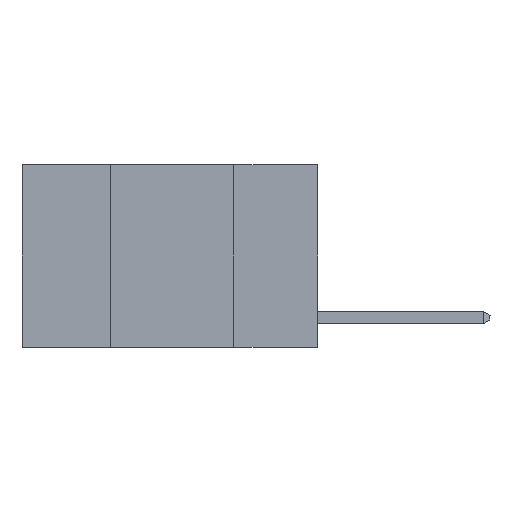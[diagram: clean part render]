
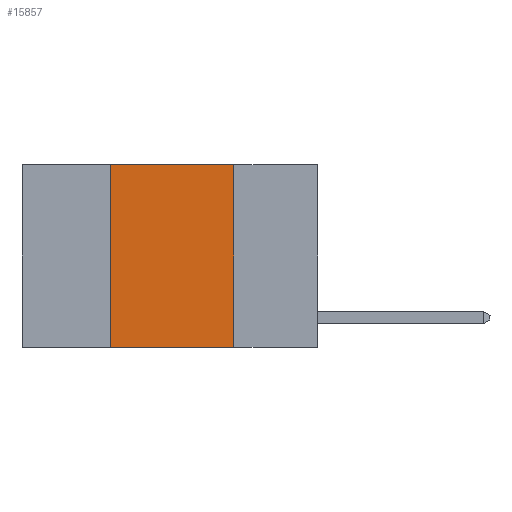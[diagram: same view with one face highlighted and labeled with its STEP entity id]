
A CAD part, left-side view. The second image highlights one B-rep face of the part: STEP entity #15857.
In plain terms, the highlighted planar face has unit normal (-1, 0, 0).
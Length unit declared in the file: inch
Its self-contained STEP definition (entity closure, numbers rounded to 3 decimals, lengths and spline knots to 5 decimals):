
#527 = FACE_OUTER_BOUND ( 'NONE', #12159, .T. ) ;
#928 = CARTESIAN_POINT ( 'NONE',  ( 0., 0.42, 0. ) ) ;
#1466 = VERTEX_POINT ( 'NONE', #21870 ) ;
#1476 = CARTESIAN_POINT ( 'NONE',  ( 0., 0.6, -0.37 ) ) ;
#1967 = VERTEX_POINT ( 'NONE', #24077 ) ;
#2682 = EDGE_CURVE ( 'NONE', #24479, #22064, #15013, .T. ) ;
#3091 = PLANE ( 'NONE',  #19471 ) ;
#3230 = DIRECTION ( 'NONE',  ( 0., 0., -1. ) ) ;
#3296 = VECTOR ( 'NONE', #20088, 39.37008 ) ;
#3658 = DIRECTION ( 'NONE',  ( 0., -1., 0. ) ) ;
#3993 = ORIENTED_EDGE ( 'NONE', *, *, #6999, .T. ) ;
#4603 = EDGE_CURVE ( 'NONE', #1967, #1466, #7291, .T. ) ;
#6799 = CARTESIAN_POINT ( 'NONE',  ( 0., 0.6, 0. ) ) ;
#6893 = DIRECTION ( 'NONE',  ( 1., 0., 0. ) ) ;
#6999 = EDGE_CURVE ( 'NONE', #1967, #22064, #16315, .T. ) ;
#7041 = CARTESIAN_POINT ( 'NONE',  ( 0., 0.17, 0. ) ) ;
#7110 = VECTOR ( 'NONE', #3230, 39.37008 ) ;
#7291 = LINE ( 'NONE', #928, #3296 ) ;
#8667 = VECTOR ( 'NONE', #3658, 39.37008 ) ;
#11179 = ORIENTED_EDGE ( 'NONE', *, *, #4603, .F. ) ;
#11641 = LINE ( 'NONE', #14410, #16242 ) ;
#12159 = EDGE_LOOP ( 'NONE', ( #19335, #12202, #11179, #3993 ) ) ;
#12202 = ORIENTED_EDGE ( 'NONE', *, *, #17796, .F. ) ;
#14410 = CARTESIAN_POINT ( 'NONE',  ( 0., 0.6, 0. ) ) ;
#15013 = LINE ( 'NONE', #15169, #7110 ) ;
#15169 = CARTESIAN_POINT ( 'NONE',  ( 0., 0.17, 0. ) ) ;
#15857 = ADVANCED_FACE ( 'NONE', ( #527 ), #3091, .F. ) ;
#16242 = VECTOR ( 'NONE', #22488, 39.37008 ) ;
#16315 = LINE ( 'NONE', #1476, #8667 ) ;
#17796 = EDGE_CURVE ( 'NONE', #1466, #24479, #11641, .T. ) ;
#19335 = ORIENTED_EDGE ( 'NONE', *, *, #2682, .F. ) ;
#19471 = AXIS2_PLACEMENT_3D ( 'NONE', #6799, #6893, #20704 ) ;
#20088 = DIRECTION ( 'NONE',  ( 0., 0., 1. ) ) ;
#20704 = DIRECTION ( 'NONE',  ( 0., 0., -1. ) ) ;
#21790 = CARTESIAN_POINT ( 'NONE',  ( 0., 0.17, -0.37 ) ) ;
#21870 = CARTESIAN_POINT ( 'NONE',  ( 0., 0.42, 0. ) ) ;
#22064 = VERTEX_POINT ( 'NONE', #21790 ) ;
#22488 = DIRECTION ( 'NONE',  ( 0., -1., 0. ) ) ;
#24077 = CARTESIAN_POINT ( 'NONE',  ( 0., 0.42, -0.37 ) ) ;
#24479 = VERTEX_POINT ( 'NONE', #7041 ) ;
